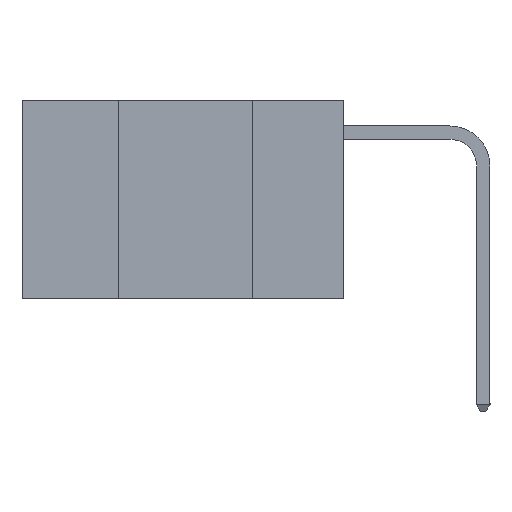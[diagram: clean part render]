
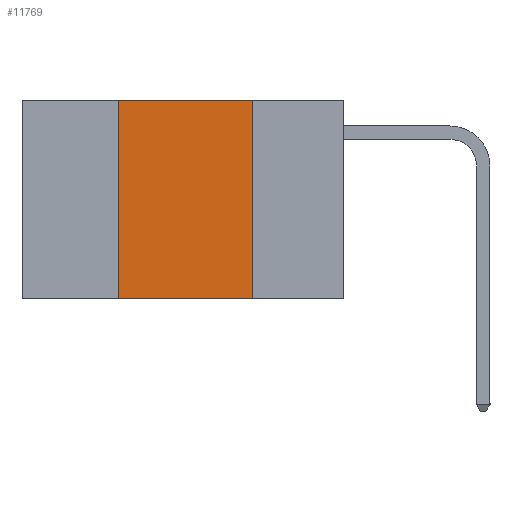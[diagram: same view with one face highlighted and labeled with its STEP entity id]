
A CAD part, left-side view. The second image highlights one B-rep face of the part: STEP entity #11769.
In plain terms, the highlighted planar face has unit normal (-1, 0, 0).
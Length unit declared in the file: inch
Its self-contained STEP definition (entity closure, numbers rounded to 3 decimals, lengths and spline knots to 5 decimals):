
#186 = CARTESIAN_POINT ( 'NONE',  ( 0., 0.42, 0. ) ) ;
#224 = CARTESIAN_POINT ( 'NONE',  ( 0., 0.17, 0. ) ) ;
#446 = CARTESIAN_POINT ( 'NONE',  ( 0., 0.6, -0.37 ) ) ;
#614 = CARTESIAN_POINT ( 'NONE',  ( 0., 0.6, 0. ) ) ;
#1481 = DIRECTION ( 'NONE',  ( 0., 0., 1. ) ) ;
#1927 = LINE ( 'NONE', #186, #5774 ) ;
#2586 = AXIS2_PLACEMENT_3D ( 'NONE', #614, #3210, #12239 ) ;
#3050 = ORIENTED_EDGE ( 'NONE', *, *, #15644, .T. ) ;
#3210 = DIRECTION ( 'NONE',  ( 1., 0., 0. ) ) ;
#3427 = DIRECTION ( 'NONE',  ( 0., -1., 0. ) ) ;
#3832 = FACE_OUTER_BOUND ( 'NONE', #11051, .T. ) ;
#4085 = CARTESIAN_POINT ( 'NONE',  ( 0., 0.42, 0. ) ) ;
#4441 = ORIENTED_EDGE ( 'NONE', *, *, #8315, .F. ) ;
#4663 = VERTEX_POINT ( 'NONE', #4928 ) ;
#4928 = CARTESIAN_POINT ( 'NONE',  ( 0., 0.17, -0.37 ) ) ;
#5320 = CARTESIAN_POINT ( 'NONE',  ( 0., 0.17, 0. ) ) ;
#5774 = VECTOR ( 'NONE', #1481, 39.37008 ) ;
#6115 = VERTEX_POINT ( 'NONE', #4085 ) ;
#6175 = VECTOR ( 'NONE', #3427, 39.37008 ) ;
#6464 = ORIENTED_EDGE ( 'NONE', *, *, #10286, .F. ) ;
#6627 = DIRECTION ( 'NONE',  ( 0., 0., -1. ) ) ;
#7241 = LINE ( 'NONE', #446, #13682 ) ;
#7319 = CARTESIAN_POINT ( 'NONE',  ( 0., 0.6, 0. ) ) ;
#8315 = EDGE_CURVE ( 'NONE', #6115, #11549, #10044, .T. ) ;
#10044 = LINE ( 'NONE', #7319, #6175 ) ;
#10286 = EDGE_CURVE ( 'NONE', #11549, #4663, #13947, .T. ) ;
#11051 = EDGE_LOOP ( 'NONE', ( #6464, #4441, #11334, #3050 ) ) ;
#11334 = ORIENTED_EDGE ( 'NONE', *, *, #13781, .F. ) ;
#11549 = VERTEX_POINT ( 'NONE', #224 ) ;
#11769 = ADVANCED_FACE ( 'NONE', ( #3832 ), #13470, .F. ) ;
#11795 = CARTESIAN_POINT ( 'NONE',  ( 0., 0.42, -0.37 ) ) ;
#12077 = DIRECTION ( 'NONE',  ( 0., -1., 0. ) ) ;
#12239 = DIRECTION ( 'NONE',  ( 0., 0., -1. ) ) ;
#13182 = VERTEX_POINT ( 'NONE', #11795 ) ;
#13195 = VECTOR ( 'NONE', #6627, 39.37008 ) ;
#13470 = PLANE ( 'NONE',  #2586 ) ;
#13682 = VECTOR ( 'NONE', #12077, 39.37008 ) ;
#13781 = EDGE_CURVE ( 'NONE', #13182, #6115, #1927, .T. ) ;
#13947 = LINE ( 'NONE', #5320, #13195 ) ;
#15644 = EDGE_CURVE ( 'NONE', #13182, #4663, #7241, .T. ) ;
